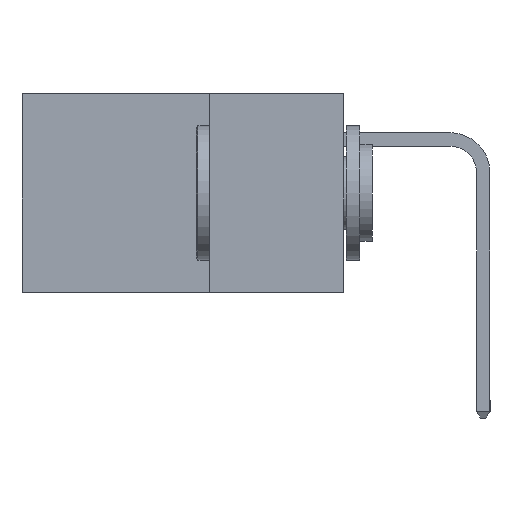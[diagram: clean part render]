
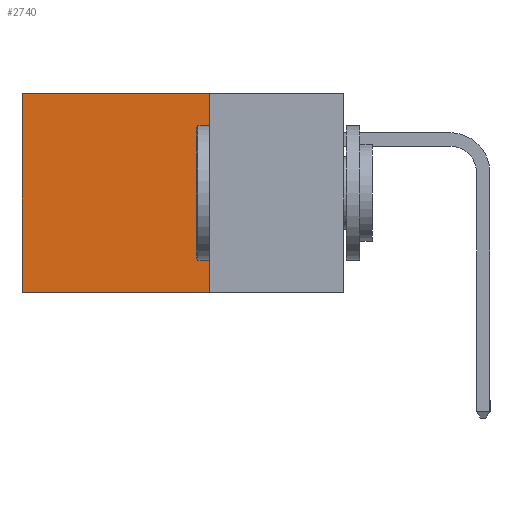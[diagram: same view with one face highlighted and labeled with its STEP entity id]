
A CAD part, left-side view. The second image highlights one B-rep face of the part: STEP entity #2740.
In plain terms, the highlighted planar face has unit normal (-1, 0, 0).
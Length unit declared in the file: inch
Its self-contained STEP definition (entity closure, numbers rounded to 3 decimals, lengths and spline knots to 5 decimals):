
#144 = CARTESIAN_POINT ( 'NONE',  ( 0.2615, 0.6, 0. ) ) ;
#275 = EDGE_CURVE ( 'NONE', #3686, #668, #4252, .T. ) ;
#295 = VECTOR ( 'NONE', #8657, 39.37008 ) ;
#587 = CARTESIAN_POINT ( 'NONE',  ( 0.2615, 0.6, -0.37 ) ) ;
#608 = EDGE_LOOP ( 'NONE', ( #2400, #2408, #2412, #2424 ) ) ;
#668 = VERTEX_POINT ( 'NONE', #144 ) ;
#1329 = VECTOR ( 'NONE', #5291, 39.37008 ) ;
#1376 = VERTEX_POINT ( 'NONE', #4802 ) ;
#1700 = VECTOR ( 'NONE', #5786, 39.37008 ) ;
#1828 = LINE ( 'NONE', #587, #6514 ) ;
#2119 = DIRECTION ( 'NONE',  ( 0., 0., -1. ) ) ;
#2168 = PLANE ( 'NONE',  #5859 ) ;
#2336 = CARTESIAN_POINT ( 'NONE',  ( 0.2615, 0.25, -0.37 ) ) ;
#2400 = ORIENTED_EDGE ( 'NONE', *, *, #7419, .T. ) ;
#2408 = ORIENTED_EDGE ( 'NONE', *, *, #10999, .F. ) ;
#2412 = ORIENTED_EDGE ( 'NONE', *, *, #9940, .F. ) ;
#2424 = ORIENTED_EDGE ( 'NONE', *, *, #275, .T. ) ;
#2450 = DIRECTION ( 'NONE',  ( 1., 0., 0. ) ) ;
#2740 = ADVANCED_FACE ( 'NONE', ( #10016 ), #2168, .F. ) ;
#3686 = VERTEX_POINT ( 'NONE', #6054 ) ;
#4252 = LINE ( 'NONE', #5635, #1700 ) ;
#4359 = CARTESIAN_POINT ( 'NONE',  ( 0.2615, 0.25, -0.37 ) ) ;
#4802 = CARTESIAN_POINT ( 'NONE',  ( 0.2615, 0.25, -0.37 ) ) ;
#5020 = VERTEX_POINT ( 'NONE', #10346 ) ;
#5291 = DIRECTION ( 'NONE',  ( 0., 1., 0. ) ) ;
#5635 = CARTESIAN_POINT ( 'NONE',  ( 0.2615, 0.25, 0. ) ) ;
#5786 = DIRECTION ( 'NONE',  ( 0., 1., 0. ) ) ;
#5859 = AXIS2_PLACEMENT_3D ( 'NONE', #2336, #2450, #2119 ) ;
#6054 = CARTESIAN_POINT ( 'NONE',  ( 0.2615, 0.25, 0. ) ) ;
#6514 = VECTOR ( 'NONE', #7118, 39.37008 ) ;
#6928 = CARTESIAN_POINT ( 'NONE',  ( 0.2615, 0.25, -0.37 ) ) ;
#7118 = DIRECTION ( 'NONE',  ( 0., 0., -1. ) ) ;
#7419 = EDGE_CURVE ( 'NONE', #668, #5020, #1828, .T. ) ;
#7714 = LINE ( 'NONE', #6928, #295 ) ;
#8657 = DIRECTION ( 'NONE',  ( 0., 0., -1. ) ) ;
#9940 = EDGE_CURVE ( 'NONE', #3686, #1376, #7714, .T. ) ;
#10016 = FACE_OUTER_BOUND ( 'NONE', #608, .T. ) ;
#10346 = CARTESIAN_POINT ( 'NONE',  ( 0.2615, 0.6, -0.37 ) ) ;
#10999 = EDGE_CURVE ( 'NONE', #1376, #5020, #11273, .T. ) ;
#11273 = LINE ( 'NONE', #4359, #1329 ) ;
